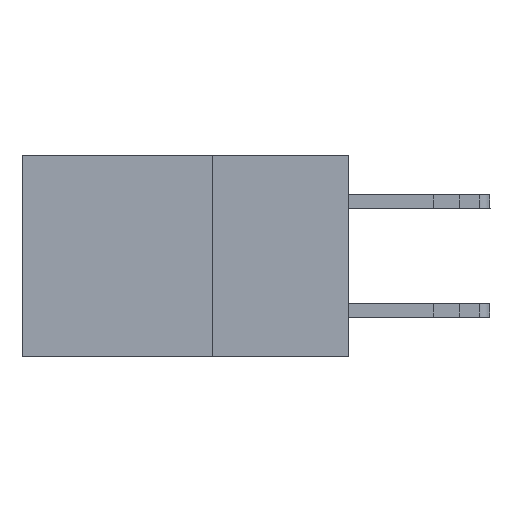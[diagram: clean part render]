
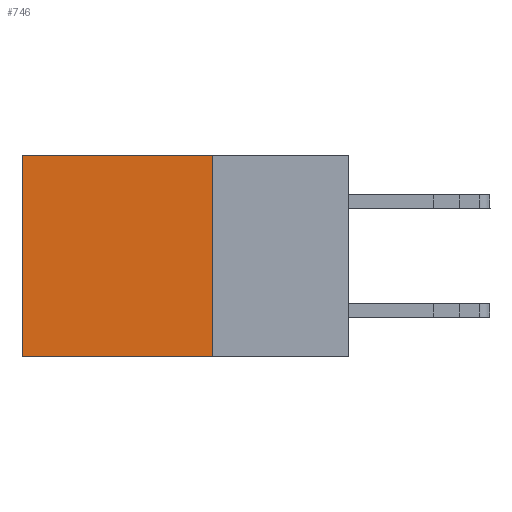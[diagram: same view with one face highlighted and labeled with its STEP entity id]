
A CAD part, left-side view. The second image highlights one B-rep face of the part: STEP entity #746.
In plain terms, the highlighted planar face has unit normal (-1, 0, 0).
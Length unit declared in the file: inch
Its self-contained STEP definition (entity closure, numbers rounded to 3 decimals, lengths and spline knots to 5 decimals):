
#25 = DIRECTION ( 'NONE',  ( 0., 0., -1. ) ) ;
#226 = FACE_OUTER_BOUND ( 'NONE', #4748, .T. ) ;
#270 = EDGE_CURVE ( 'NONE', #11064, #7986, #10597, .T. ) ;
#746 = ADVANCED_FACE ( 'NONE', ( #226 ), #4976, .F. ) ;
#1108 = CARTESIAN_POINT ( 'NONE',  ( 0.2615, 0.6, -0.37 ) ) ;
#1899 = LINE ( 'NONE', #2966, #8096 ) ;
#2966 = CARTESIAN_POINT ( 'NONE',  ( 0.2615, 0.25, -0.37 ) ) ;
#3040 = ORIENTED_EDGE ( 'NONE', *, *, #8687, .F. ) ;
#3548 = VECTOR ( 'NONE', #5857, 39.37008 ) ;
#3567 = VERTEX_POINT ( 'NONE', #7688 ) ;
#3848 = ORIENTED_EDGE ( 'NONE', *, *, #4672, .T. ) ;
#4672 = EDGE_CURVE ( 'NONE', #11162, #11064, #6751, .T. ) ;
#4748 = EDGE_LOOP ( 'NONE', ( #8735, #9840, #3040, #3848 ) ) ;
#4789 = CARTESIAN_POINT ( 'NONE',  ( 0.2615, 0.25, 0. ) ) ;
#4976 = PLANE ( 'NONE',  #7143 ) ;
#5857 = DIRECTION ( 'NONE',  ( 0., 1., 0. ) ) ;
#6751 = LINE ( 'NONE', #4789, #3548 ) ;
#7011 = DIRECTION ( 'NONE',  ( 0., 0., -1. ) ) ;
#7143 = AXIS2_PLACEMENT_3D ( 'NONE', #8817, #10787, #7011 ) ;
#7688 = CARTESIAN_POINT ( 'NONE',  ( 0.2615, 0.25, -0.37 ) ) ;
#7986 = VERTEX_POINT ( 'NONE', #9210 ) ;
#8096 = VECTOR ( 'NONE', #8894, 39.37008 ) ;
#8289 = EDGE_CURVE ( 'NONE', #3567, #7986, #1899, .T. ) ;
#8685 = CARTESIAN_POINT ( 'NONE',  ( 0.2615, 0.25, -0.37 ) ) ;
#8687 = EDGE_CURVE ( 'NONE', #11162, #3567, #8750, .T. ) ;
#8735 = ORIENTED_EDGE ( 'NONE', *, *, #270, .T. ) ;
#8750 = LINE ( 'NONE', #8685, #11120 ) ;
#8817 = CARTESIAN_POINT ( 'NONE',  ( 0.2615, 0.25, -0.37 ) ) ;
#8874 = DIRECTION ( 'NONE',  ( 0., 0., -1. ) ) ;
#8894 = DIRECTION ( 'NONE',  ( 0., 1., 0. ) ) ;
#9210 = CARTESIAN_POINT ( 'NONE',  ( 0.2615, 0.6, -0.37 ) ) ;
#9593 = CARTESIAN_POINT ( 'NONE',  ( 0.2615, 0.6, 0. ) ) ;
#9840 = ORIENTED_EDGE ( 'NONE', *, *, #8289, .F. ) ;
#9982 = CARTESIAN_POINT ( 'NONE',  ( 0.2615, 0.25, 0. ) ) ;
#9990 = VECTOR ( 'NONE', #8874, 39.37008 ) ;
#10597 = LINE ( 'NONE', #1108, #9990 ) ;
#10787 = DIRECTION ( 'NONE',  ( 1., 0., 0. ) ) ;
#11064 = VERTEX_POINT ( 'NONE', #9593 ) ;
#11120 = VECTOR ( 'NONE', #25, 39.37008 ) ;
#11162 = VERTEX_POINT ( 'NONE', #9982 ) ;
